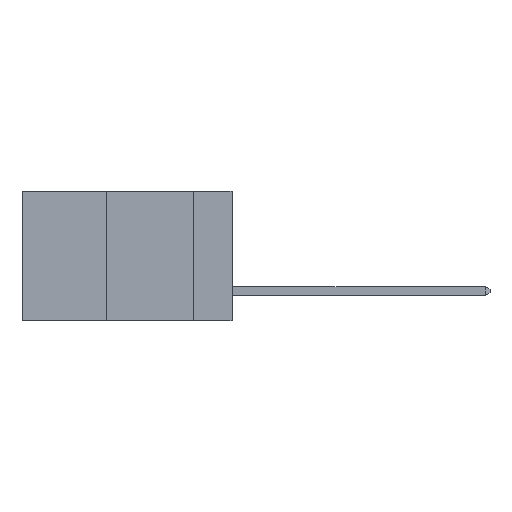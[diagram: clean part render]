
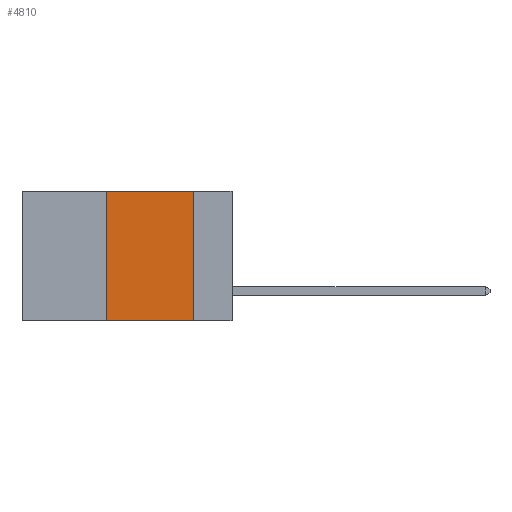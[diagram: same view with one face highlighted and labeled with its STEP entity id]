
A CAD part, left-side view. The second image highlights one B-rep face of the part: STEP entity #4810.
In plain terms, the highlighted planar face has unit normal (-1, 0, 0).
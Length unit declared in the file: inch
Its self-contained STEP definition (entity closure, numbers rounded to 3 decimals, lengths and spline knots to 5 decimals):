
#112 = CARTESIAN_POINT ( 'NONE',  ( 0., 0.11, 0. ) ) ;
#581 = DIRECTION ( 'NONE',  ( 0., 0., -1. ) ) ;
#1571 = EDGE_CURVE ( 'NONE', #15701, #4955, #19949, .T. ) ;
#2527 = AXIS2_PLACEMENT_3D ( 'NONE', #23483, #17817, #581 ) ;
#4141 = CARTESIAN_POINT ( 'NONE',  ( 0., 0.11, -0.37 ) ) ;
#4736 = CARTESIAN_POINT ( 'NONE',  ( 0., 0.6, 0. ) ) ;
#4810 = ADVANCED_FACE ( 'NONE', ( #21187 ), #14943, .F. ) ;
#4955 = VERTEX_POINT ( 'NONE', #4141 ) ;
#5247 = CARTESIAN_POINT ( 'NONE',  ( 0., 0.36, -0.37 ) ) ;
#5545 = LINE ( 'NONE', #8328, #19943 ) ;
#5900 = DIRECTION ( 'NONE',  ( 0., 0., -1. ) ) ;
#6607 = LINE ( 'NONE', #4736, #35231 ) ;
#8328 = CARTESIAN_POINT ( 'NONE',  ( 0., 0.36, 0. ) ) ;
#8567 = EDGE_CURVE ( 'NONE', #33416, #4955, #22623, .T. ) ;
#10264 = ORIENTED_EDGE ( 'NONE', *, *, #28507, .F. ) ;
#11760 = ORIENTED_EDGE ( 'NONE', *, *, #8567, .F. ) ;
#13542 = ORIENTED_EDGE ( 'NONE', *, *, #19438, .F. ) ;
#14897 = DIRECTION ( 'NONE',  ( 0., -1., 0. ) ) ;
#14943 = PLANE ( 'NONE',  #2527 ) ;
#15701 = VERTEX_POINT ( 'NONE', #5247 ) ;
#17817 = DIRECTION ( 'NONE',  ( 1., 0., 0. ) ) ;
#19064 = VECTOR ( 'NONE', #14897, 39.37008 ) ;
#19438 = EDGE_CURVE ( 'NONE', #15701, #29571, #5545, .T. ) ;
#19765 = DIRECTION ( 'NONE',  ( 0., 0., 1. ) ) ;
#19943 = VECTOR ( 'NONE', #19765, 39.37008 ) ;
#19949 = LINE ( 'NONE', #20658, #19064 ) ;
#20658 = CARTESIAN_POINT ( 'NONE',  ( 0., 0.6, -0.37 ) ) ;
#21187 = FACE_OUTER_BOUND ( 'NONE', #36792, .T. ) ;
#21935 = ORIENTED_EDGE ( 'NONE', *, *, #1571, .T. ) ;
#22623 = LINE ( 'NONE', #112, #36838 ) ;
#23483 = CARTESIAN_POINT ( 'NONE',  ( 0., 0.6, 0. ) ) ;
#27617 = DIRECTION ( 'NONE',  ( 0., -1., 0. ) ) ;
#28507 = EDGE_CURVE ( 'NONE', #29571, #33416, #6607, .T. ) ;
#29571 = VERTEX_POINT ( 'NONE', #32542 ) ;
#32542 = CARTESIAN_POINT ( 'NONE',  ( 0., 0.36, 0. ) ) ;
#32928 = CARTESIAN_POINT ( 'NONE',  ( 0., 0.11, 0. ) ) ;
#33416 = VERTEX_POINT ( 'NONE', #32928 ) ;
#35231 = VECTOR ( 'NONE', #27617, 39.37008 ) ;
#36792 = EDGE_LOOP ( 'NONE', ( #11760, #10264, #13542, #21935 ) ) ;
#36838 = VECTOR ( 'NONE', #5900, 39.37008 ) ;
